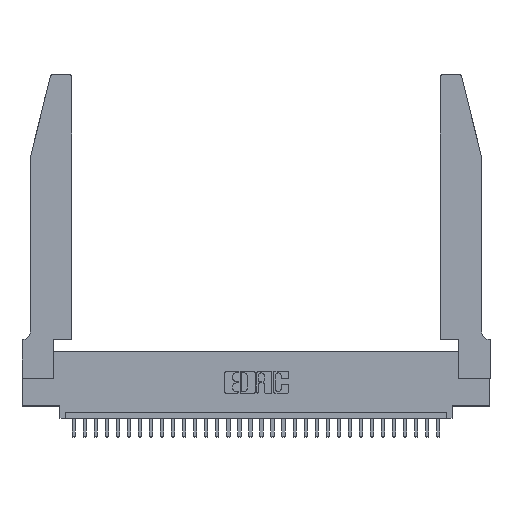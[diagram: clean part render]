
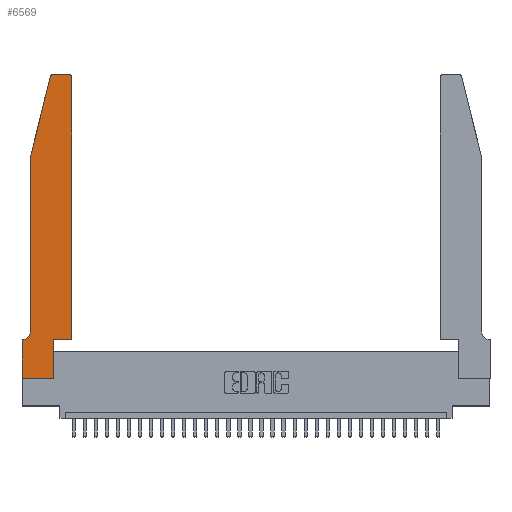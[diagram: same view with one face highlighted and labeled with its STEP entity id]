
A CAD part, top view. The second image highlights one B-rep face of the part: STEP entity #6569.
In plain terms, the highlighted planar face has unit normal (0, 0, 1).
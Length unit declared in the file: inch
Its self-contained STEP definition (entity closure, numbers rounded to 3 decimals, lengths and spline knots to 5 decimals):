
#336 = EDGE_CURVE ( 'NONE', #5408, #24941, #5308, .T. ) ;
#704 = ORIENTED_EDGE ( 'NONE', *, *, #2084, .T. ) ;
#776 = DIRECTION ( 'NONE',  ( -1., 0., 0. ) ) ;
#811 = CARTESIAN_POINT ( 'NONE',  ( 0., 0., 0.37 ) ) ;
#1094 = CARTESIAN_POINT ( 'NONE',  ( 0.284, 2.72, 0.37 ) ) ;
#1099 = VECTOR ( 'NONE', #30677, 39.37008 ) ;
#1171 = EDGE_CURVE ( 'NONE', #24941, #12372, #15525, .T. ) ;
#1203 = VECTOR ( 'NONE', #15734, 39.37008 ) ;
#2084 = EDGE_CURVE ( 'NONE', #24739, #21483, #8632, .T. ) ;
#2498 = CARTESIAN_POINT ( 'NONE',  ( 0.0755, 0.42, 0.37 ) ) ;
#2698 = LINE ( 'NONE', #21641, #20296 ) ;
#3225 = CARTESIAN_POINT ( 'NONE',  ( 0.284, 2.75, 0.37 ) ) ;
#3393 = CARTESIAN_POINT ( 'NONE',  ( 0.0755, 2., 0.37 ) ) ;
#4225 = DIRECTION ( 'NONE',  ( 1., 0., 0. ) ) ;
#5093 = EDGE_CURVE ( 'NONE', #31366, #30060, #7964, .T. ) ;
#5308 = LINE ( 'NONE', #17880, #1099 ) ;
#5408 = VERTEX_POINT ( 'NONE', #24494 ) ;
#6569 = ADVANCED_FACE ( 'NONE', ( #10547 ), #29542, .T. ) ;
#6717 = AXIS2_PLACEMENT_3D ( 'NONE', #13695, #11574, #4225 ) ;
#6754 = VERTEX_POINT ( 'NONE', #30396 ) ;
#6767 = VECTOR ( 'NONE', #7095, 39.37008 ) ;
#6964 = LINE ( 'NONE', #16895, #23373 ) ;
#7095 = DIRECTION ( 'NONE',  ( -1., 0., 0. ) ) ;
#7573 = AXIS2_PLACEMENT_3D ( 'NONE', #12823, #22751, #776 ) ;
#7618 = DIRECTION ( 'NONE',  ( 0., 0., 1. ) ) ;
#7964 = CIRCLE ( 'NONE', #12219, 0.03 ) ;
#8481 = CARTESIAN_POINT ( 'NONE',  ( 0.25487, 2.72718, 0.37 ) ) ;
#8632 = LINE ( 'NONE', #24684, #6767 ) ;
#8883 = VERTEX_POINT ( 'NONE', #811 ) ;
#9106 = VERTEX_POINT ( 'NONE', #18612 ) ;
#9125 = CARTESIAN_POINT ( 'NONE',  ( 0.2865, 0., 0.37 ) ) ;
#9575 = DIRECTION ( 'NONE',  ( 1., 0., 0. ) ) ;
#9582 = DIRECTION ( 'NONE',  ( -0.239, -0.971, 0. ) ) ;
#9743 = CARTESIAN_POINT ( 'NONE',  ( 0.4505, 2.72, 0.37 ) ) ;
#9952 = LINE ( 'NONE', #21959, #25642 ) ;
#10072 = DIRECTION ( 'NONE',  ( 1., 0., 0. ) ) ;
#10129 = VERTEX_POINT ( 'NONE', #2498 ) ;
#10547 = FACE_OUTER_BOUND ( 'NONE', #15268, .T. ) ;
#10596 = EDGE_CURVE ( 'NONE', #9106, #5408, #10714, .T. ) ;
#10714 = LINE ( 'NONE', #29677, #28325 ) ;
#11574 = DIRECTION ( 'NONE',  ( 0., 0., 1. ) ) ;
#12219 = AXIS2_PLACEMENT_3D ( 'NONE', #1094, #27928, #13246 ) ;
#12274 = ORIENTED_EDGE ( 'NONE', *, *, #336, .T. ) ;
#12372 = VERTEX_POINT ( 'NONE', #14749 ) ;
#12823 = CARTESIAN_POINT ( 'NONE',  ( 0.0055, 0.42, 0.37 ) ) ;
#13246 = DIRECTION ( 'NONE',  ( 1., 0., 0. ) ) ;
#13695 = CARTESIAN_POINT ( 'NONE',  ( 0.4205, 2.72, 0.37 ) ) ;
#14280 = CARTESIAN_POINT ( 'NONE',  ( 0.2605, 2.75, 0.37 ) ) ;
#14456 = EDGE_CURVE ( 'NONE', #12372, #31366, #16408, .T. ) ;
#14749 = CARTESIAN_POINT ( 'NONE',  ( 0.4205, 2.75, 0.37 ) ) ;
#14769 = ORIENTED_EDGE ( 'NONE', *, *, #19618, .T. ) ;
#14795 = ORIENTED_EDGE ( 'NONE', *, *, #20165, .T. ) ;
#14853 = CARTESIAN_POINT ( 'NONE',  ( 0., 0.35, 0.37 ) ) ;
#14986 = DIRECTION ( 'NONE',  ( 1., 0., 0. ) ) ;
#15268 = EDGE_LOOP ( 'NONE', ( #20712, #29551, #14769, #26075, #31134, #704, #22848, #14795, #22980, #28388, #12274, #28378 ) ) ;
#15525 = CIRCLE ( 'NONE', #6717, 0.03 ) ;
#15734 = DIRECTION ( 'NONE',  ( 0., -1., 0. ) ) ;
#16408 = LINE ( 'NONE', #14280, #26402 ) ;
#16895 = CARTESIAN_POINT ( 'NONE',  ( 0., 0., 0.37 ) ) ;
#17880 = CARTESIAN_POINT ( 'NONE',  ( 0.4505, 0.35, 0.37 ) ) ;
#18028 = CIRCLE ( 'NONE', #7573, 0.07 ) ;
#18315 = EDGE_CURVE ( 'NONE', #10129, #24739, #18028, .T. ) ;
#18612 = CARTESIAN_POINT ( 'NONE',  ( 0.2865, 0.35, 0.37 ) ) ;
#18944 = CARTESIAN_POINT ( 'NONE',  ( 0., 0.35, 0.37 ) ) ;
#19618 = EDGE_CURVE ( 'NONE', #30060, #6754, #2698, .T. ) ;
#20069 = DIRECTION ( 'NONE',  ( 0., 1., 0. ) ) ;
#20165 = EDGE_CURVE ( 'NONE', #8883, #25014, #9952, .T. ) ;
#20296 = VECTOR ( 'NONE', #9582, 39.37008 ) ;
#20689 = LINE ( 'NONE', #3393, #1203 ) ;
#20712 = ORIENTED_EDGE ( 'NONE', *, *, #14456, .T. ) ;
#21483 = VERTEX_POINT ( 'NONE', #18944 ) ;
#21641 = CARTESIAN_POINT ( 'NONE',  ( 0.0755, 2., 0.37 ) ) ;
#21959 = CARTESIAN_POINT ( 'NONE',  ( 0., 0., 0.37 ) ) ;
#21992 = LINE ( 'NONE', #27073, #28526 ) ;
#22751 = DIRECTION ( 'NONE',  ( 0., 0., -1. ) ) ;
#22848 = ORIENTED_EDGE ( 'NONE', *, *, #30220, .T. ) ;
#22980 = ORIENTED_EDGE ( 'NONE', *, *, #27262, .T. ) ;
#23373 = VECTOR ( 'NONE', #24205, 39.37008 ) ;
#24205 = DIRECTION ( 'NONE',  ( 0., -1., 0. ) ) ;
#24406 = AXIS2_PLACEMENT_3D ( 'NONE', #14853, #7618, #10072 ) ;
#24494 = CARTESIAN_POINT ( 'NONE',  ( 0.4505, 0.35, 0.37 ) ) ;
#24684 = CARTESIAN_POINT ( 'NONE',  ( 0.0755, 0.35, 0.37 ) ) ;
#24739 = VERTEX_POINT ( 'NONE', #26843 ) ;
#24941 = VERTEX_POINT ( 'NONE', #9743 ) ;
#25014 = VERTEX_POINT ( 'NONE', #9125 ) ;
#25642 = VECTOR ( 'NONE', #9575, 39.37008 ) ;
#26075 = ORIENTED_EDGE ( 'NONE', *, *, #29997, .T. ) ;
#26402 = VECTOR ( 'NONE', #31245, 39.37008 ) ;
#26843 = CARTESIAN_POINT ( 'NONE',  ( 0.0055, 0.35, 0.37 ) ) ;
#27073 = CARTESIAN_POINT ( 'NONE',  ( 0.2865, 0.35, 0.37 ) ) ;
#27262 = EDGE_CURVE ( 'NONE', #25014, #9106, #21992, .T. ) ;
#27928 = DIRECTION ( 'NONE',  ( 0., 0., 1. ) ) ;
#28325 = VECTOR ( 'NONE', #14986, 39.37008 ) ;
#28378 = ORIENTED_EDGE ( 'NONE', *, *, #1171, .T. ) ;
#28388 = ORIENTED_EDGE ( 'NONE', *, *, #10596, .T. ) ;
#28526 = VECTOR ( 'NONE', #20069, 39.37008 ) ;
#29542 = PLANE ( 'NONE',  #24406 ) ;
#29551 = ORIENTED_EDGE ( 'NONE', *, *, #5093, .T. ) ;
#29677 = CARTESIAN_POINT ( 'NONE',  ( 0.4505, 0.35, 0.37 ) ) ;
#29997 = EDGE_CURVE ( 'NONE', #6754, #10129, #20689, .T. ) ;
#30060 = VERTEX_POINT ( 'NONE', #8481 ) ;
#30220 = EDGE_CURVE ( 'NONE', #21483, #8883, #6964, .T. ) ;
#30396 = CARTESIAN_POINT ( 'NONE',  ( 0.0755, 2., 0.37 ) ) ;
#30677 = DIRECTION ( 'NONE',  ( 0., 1., 0. ) ) ;
#31134 = ORIENTED_EDGE ( 'NONE', *, *, #18315, .T. ) ;
#31245 = DIRECTION ( 'NONE',  ( -1., 0., 0. ) ) ;
#31366 = VERTEX_POINT ( 'NONE', #3225 ) ;
